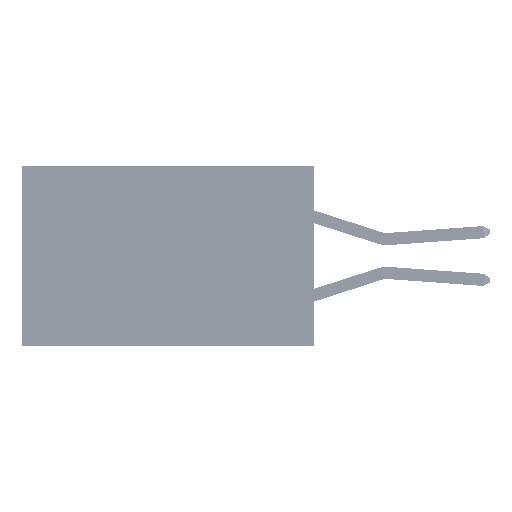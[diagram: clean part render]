
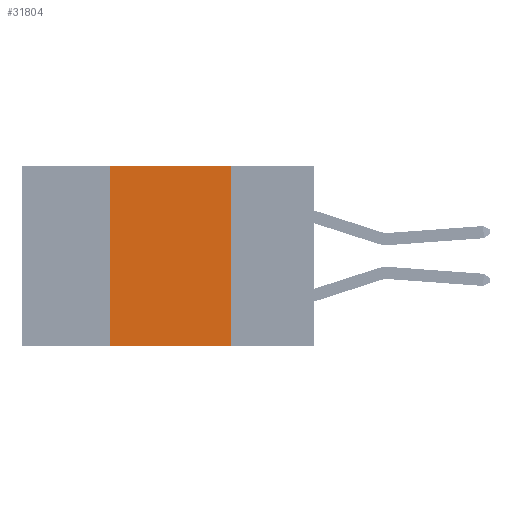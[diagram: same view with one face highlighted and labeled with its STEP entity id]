
A CAD part, left-side view. The second image highlights one B-rep face of the part: STEP entity #31804.
In plain terms, the highlighted planar face has unit normal (-1, 0, 0).
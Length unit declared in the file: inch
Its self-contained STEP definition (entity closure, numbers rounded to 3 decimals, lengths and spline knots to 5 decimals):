
#162 = EDGE_CURVE ( 'NONE', #18242, #5447, #40345, .T. ) ;
#788 = DIRECTION ( 'NONE',  ( 0., -1., 0. ) ) ;
#2050 = DIRECTION ( 'NONE',  ( 0., -1., 0. ) ) ;
#2342 = ORIENTED_EDGE ( 'NONE', *, *, #162, .F. ) ;
#2836 = VECTOR ( 'NONE', #32451, 39.37008 ) ;
#2941 = DIRECTION ( 'NONE',  ( 0., 0., 1. ) ) ;
#5447 = VERTEX_POINT ( 'NONE', #37380 ) ;
#8689 = EDGE_CURVE ( 'NONE', #37228, #38421, #16092, .T. ) ;
#9954 = EDGE_CURVE ( 'NONE', #18242, #38421, #33522, .T. ) ;
#11490 = DIRECTION ( 'NONE',  ( 0., 0., -1. ) ) ;
#11660 = PLANE ( 'NONE',  #49458 ) ;
#11835 = ORIENTED_EDGE ( 'NONE', *, *, #21331, .F. ) ;
#14251 = CARTESIAN_POINT ( 'NONE',  ( 0., 0.42, 0. ) ) ;
#16092 = LINE ( 'NONE', #32292, #2836 ) ;
#18242 = VERTEX_POINT ( 'NONE', #20870 ) ;
#19734 = CARTESIAN_POINT ( 'NONE',  ( 0., 0.6, 0. ) ) ;
#20870 = CARTESIAN_POINT ( 'NONE',  ( 0., 0.42, -0.37 ) ) ;
#21223 = ORIENTED_EDGE ( 'NONE', *, *, #8689, .F. ) ;
#21331 = EDGE_CURVE ( 'NONE', #5447, #37228, #28007, .T. ) ;
#24680 = VECTOR ( 'NONE', #2941, 39.37008 ) ;
#28007 = LINE ( 'NONE', #40025, #46120 ) ;
#29418 = ORIENTED_EDGE ( 'NONE', *, *, #9954, .T. ) ;
#29743 = CARTESIAN_POINT ( 'NONE',  ( 0., 0.17, -0.37 ) ) ;
#30240 = FACE_OUTER_BOUND ( 'NONE', #31881, .T. ) ;
#31804 = ADVANCED_FACE ( 'NONE', ( #30240 ), #11660, .F. ) ;
#31881 = EDGE_LOOP ( 'NONE', ( #21223, #11835, #2342, #29418 ) ) ;
#31883 = CARTESIAN_POINT ( 'NONE',  ( 0., 0.17, 0. ) ) ;
#32292 = CARTESIAN_POINT ( 'NONE',  ( 0., 0.17, 0. ) ) ;
#32324 = VECTOR ( 'NONE', #788, 39.37008 ) ;
#32451 = DIRECTION ( 'NONE',  ( 0., 0., -1. ) ) ;
#33522 = LINE ( 'NONE', #47228, #32324 ) ;
#37228 = VERTEX_POINT ( 'NONE', #31883 ) ;
#37380 = CARTESIAN_POINT ( 'NONE',  ( 0., 0.42, 0. ) ) ;
#38421 = VERTEX_POINT ( 'NONE', #29743 ) ;
#40025 = CARTESIAN_POINT ( 'NONE',  ( 0., 0.6, 0. ) ) ;
#40345 = LINE ( 'NONE', #14251, #24680 ) ;
#46105 = DIRECTION ( 'NONE',  ( 1., 0., 0. ) ) ;
#46120 = VECTOR ( 'NONE', #2050, 39.37008 ) ;
#47228 = CARTESIAN_POINT ( 'NONE',  ( 0., 0.6, -0.37 ) ) ;
#49458 = AXIS2_PLACEMENT_3D ( 'NONE', #19734, #46105, #11490 ) ;
